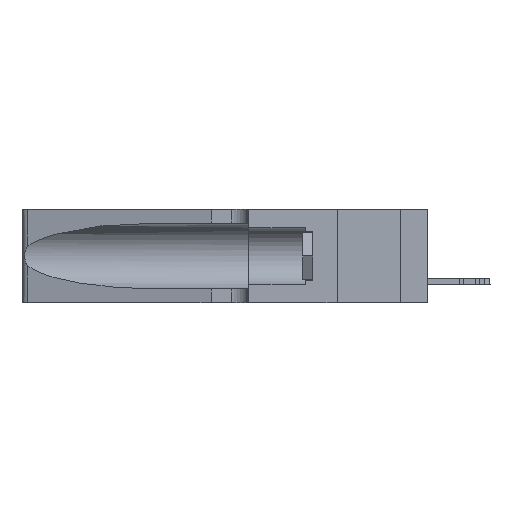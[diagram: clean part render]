
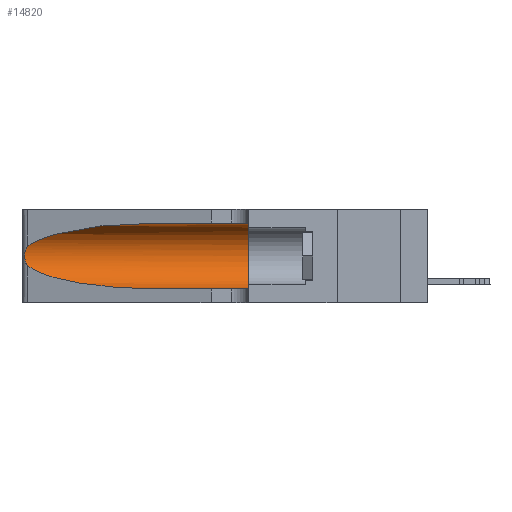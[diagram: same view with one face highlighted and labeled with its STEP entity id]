
A CAD part, left-side view. The second image highlights one B-rep face of the part: STEP entity #14820.
In plain terms, the highlighted cylindrical face has radius 3.308 mm (diameter 6.617 mm), a partial arc.
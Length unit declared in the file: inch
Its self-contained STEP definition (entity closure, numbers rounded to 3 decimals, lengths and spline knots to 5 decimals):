
#420 = CARTESIAN_POINT ( 'NONE',  ( 0.1305, 1.61858, 0.05475 ) ) ;
#620 = VERTEX_POINT ( 'NONE', #20498 ) ;
#1757 = B_SPLINE_CURVE_WITH_KNOTS ( 'NONE', 3,
 ( #44314, #40384, #38063, #34540, #30437, #20017, #2328, #45249, #44948, #41546, #20160, #9062, #34220, #9391 ),
 .UNSPECIFIED., .F., .F.,
 ( 4, 2, 2, 2, 2, 2, 4 ),
 ( 0., 0.00027, 0.00053, 0.00107, 0.0016, 0.00187, 0.00214 ),
 .UNSPECIFIED. ) ;
#1828 = EDGE_CURVE ( 'NONE', #620, #30842, #43221, .T. ) ;
#2328 = CARTESIAN_POINT ( 'NONE',  ( 0.26075, 1.23896, 0.19203 ) ) ;
#4361 = EDGE_CURVE ( 'NONE', #33025, #15079, #32147, .T. ) ;
#4753 = LINE ( 'NONE', #420, #41095 ) ;
#5808 = CARTESIAN_POINT ( 'NONE',  ( 0.18966, 0.96281, 0.05475 ) ) ;
#8367 = CARTESIAN_POINT ( 'NONE',  ( 0.1305, 0.72297, 0.05475 ) ) ;
#8808 = CARTESIAN_POINT ( 'NONE',  ( 0.25487, 1.22718, 0.14631 ) ) ;
#8922 = CARTESIAN_POINT ( 'NONE',  ( 0.2373, 1.15595, 0.08982 ) ) ;
#9062 = CARTESIAN_POINT ( 'NONE',  ( 0.25639, 1.23186, 0.15144 ) ) ;
#9391 = CARTESIAN_POINT ( 'NONE',  ( 0.25487, 1.22718, 0.14631 ) ) ;
#11127 = LINE ( 'NONE', #15389, #13423 ) ;
#11323 = ORIENTED_EDGE ( 'NONE', *, *, #30430, .T. ) ;
#13423 = VECTOR ( 'NONE', #22605, 39.37008 ) ;
#14820 = ADVANCED_FACE ( 'NONE', ( #25134 ), #34073, .F. ) ;
#15079 = VERTEX_POINT ( 'NONE', #26498 ) ;
#15389 = CARTESIAN_POINT ( 'NONE',  ( 0.1305, 1.61858, 0.31525 ) ) ;
#17266 = CARTESIAN_POINT ( 'NONE',  ( 0.18966, 0.96281, 0.31525 ) ) ;
#17792 = DIRECTION ( 'NONE',  ( 0., 1., 0. ) ) ;
#17944 = DIRECTION ( 'NONE',  ( 0., 0., 1. ) ) ;
#18574 = ORIENTED_EDGE ( 'NONE', *, *, #4361, .T. ) ;
#20017 = CARTESIAN_POINT ( 'NONE',  ( 0.26018, 1.23835, 0.19895 ) ) ;
#20160 = CARTESIAN_POINT ( 'NONE',  ( 0.25789, 1.23486, 0.15765 ) ) ;
#20498 = CARTESIAN_POINT ( 'NONE',  ( 0.1305, 0.72297, 0.31525 ) ) ;
#22605 = DIRECTION ( 'NONE',  ( 0., -1., 0. ) ) ;
#25119 = DIRECTION ( 'NONE',  ( 0., -1., 0. ) ) ;
#25134 = FACE_OUTER_BOUND ( 'NONE', #42248, .T. ) ;
#25412 = VERTEX_POINT ( 'NONE', #39719 ) ;
#26498 = CARTESIAN_POINT ( 'NONE',  ( 0.1305, 0.72297, 0.05475 ) ) ;
#27820 = CIRCLE ( 'NONE', #44158, 0.13025 ) ;
#28019 = CARTESIAN_POINT ( 'NONE',  ( 0.2373, 1.15595, 0.28018 ) ) ;
#28172 = DIRECTION ( 'NONE',  ( 0., -1., 0. ) ) ;
#28261 = CARTESIAN_POINT ( 'NONE',  ( 0.1305, 0.35, 0.185 ) ) ;
#29312 = ORIENTED_EDGE ( 'NONE', *, *, #42139, .F. ) ;
#30430 = EDGE_CURVE ( 'NONE', #30842, #33025, #1757, .T. ) ;
#30437 = CARTESIAN_POINT ( 'NONE',  ( 0.25854, 1.2359, 0.20912 ) ) ;
#30842 = VERTEX_POINT ( 'NONE', #43828 ) ;
#31943 = CARTESIAN_POINT ( 'NONE',  ( 0.25487, 1.22718, 0.22369 ) ) ;
#32147 =( BOUNDED_CURVE ( )  B_SPLINE_CURVE ( 3, ( #40895, #8922, #5808, #8367 ),
 .UNSPECIFIED., .F., .F. ) 
 B_SPLINE_CURVE_WITH_KNOTS ( ( 4, 4 ),
 ( 3.44316, 4.71239 ),
 .UNSPECIFIED. ) 
 CURVE ( )  GEOMETRIC_REPRESENTATION_ITEM ( )  RATIONAL_B_SPLINE_CURVE ( ( 1., 0.87, 0.87, 1. ) ) 
 REPRESENTATION_ITEM ( '' )  );
#33025 = VERTEX_POINT ( 'NONE', #8808 ) ;
#33332 = VERTEX_POINT ( 'NONE', #35924 ) ;
#34073 = CYLINDRICAL_SURFACE ( 'NONE', #42857, 0.13025 ) ;
#34220 = CARTESIAN_POINT ( 'NONE',  ( 0.25555, 1.22993, 0.14849 ) ) ;
#34540 = CARTESIAN_POINT ( 'NONE',  ( 0.25787, 1.23484, 0.2124 ) ) ;
#35028 = EDGE_CURVE ( 'NONE', #15079, #33332, #4753, .T. ) ;
#35040 = ORIENTED_EDGE ( 'NONE', *, *, #35028, .T. ) ;
#35669 = DIRECTION ( 'NONE',  ( 0., 0., -1. ) ) ;
#35924 = CARTESIAN_POINT ( 'NONE',  ( 0.1305, 0.35, 0.05475 ) ) ;
#38063 = CARTESIAN_POINT ( 'NONE',  ( 0.25639, 1.23184, 0.21858 ) ) ;
#38293 = ORIENTED_EDGE ( 'NONE', *, *, #43199, .F. ) ;
#39216 = CARTESIAN_POINT ( 'NONE',  ( 0.1305, 0.72297, 0.31525 ) ) ;
#39319 = CARTESIAN_POINT ( 'NONE',  ( 0.1305, 1.61858, 0.185 ) ) ;
#39719 = CARTESIAN_POINT ( 'NONE',  ( 0.1305, 0.35, 0.31525 ) ) ;
#40384 = CARTESIAN_POINT ( 'NONE',  ( 0.25555, 1.22994, 0.2215 ) ) ;
#40895 = CARTESIAN_POINT ( 'NONE',  ( 0.25487, 1.22718, 0.14631 ) ) ;
#41095 = VECTOR ( 'NONE', #25119, 39.37008 ) ;
#41546 = CARTESIAN_POINT ( 'NONE',  ( 0.25856, 1.23593, 0.16098 ) ) ;
#41758 = ORIENTED_EDGE ( 'NONE', *, *, #1828, .T. ) ;
#42139 = EDGE_CURVE ( 'NONE', #620, #25412, #11127, .T. ) ;
#42248 = EDGE_LOOP ( 'NONE', ( #41758, #11323, #18574, #35040, #38293, #29312 ) ) ;
#42857 = AXIS2_PLACEMENT_3D ( 'NONE', #39319, #28172, #35669 ) ;
#43199 = EDGE_CURVE ( 'NONE', #25412, #33332, #27820, .T. ) ;
#43221 =( BOUNDED_CURVE ( )  B_SPLINE_CURVE ( 3, ( #39216, #17266, #28019, #31943 ),
 .UNSPECIFIED., .F., .F. ) 
 B_SPLINE_CURVE_WITH_KNOTS ( ( 4, 4 ),
 ( 1.5708, 2.84003 ),
 .UNSPECIFIED. ) 
 CURVE ( )  GEOMETRIC_REPRESENTATION_ITEM ( )  RATIONAL_B_SPLINE_CURVE ( ( 1., 0.87, 0.87, 1. ) ) 
 REPRESENTATION_ITEM ( '' )  );
#43828 = CARTESIAN_POINT ( 'NONE',  ( 0.25487, 1.22718, 0.22369 ) ) ;
#44158 = AXIS2_PLACEMENT_3D ( 'NONE', #28261, #17792, #17944 ) ;
#44314 = CARTESIAN_POINT ( 'NONE',  ( 0.25487, 1.22718, 0.22369 ) ) ;
#44948 = CARTESIAN_POINT ( 'NONE',  ( 0.26017, 1.23833, 0.17102 ) ) ;
#45249 = CARTESIAN_POINT ( 'NONE',  ( 0.26075, 1.23896, 0.178 ) ) ;
